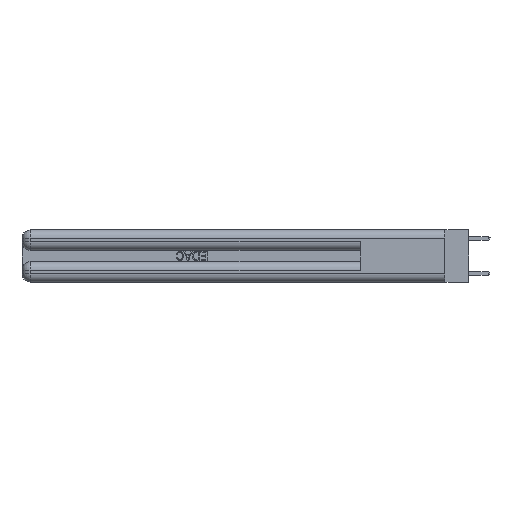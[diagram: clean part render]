
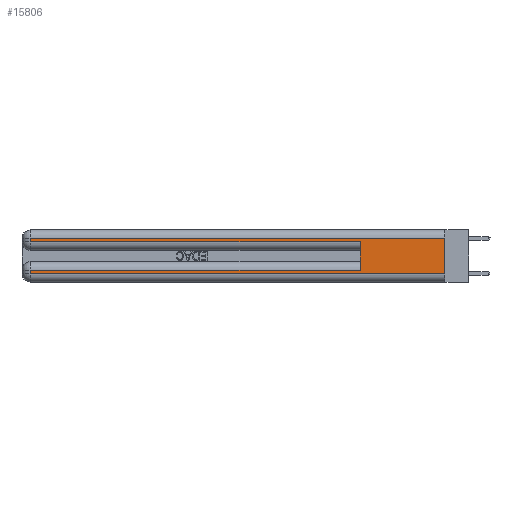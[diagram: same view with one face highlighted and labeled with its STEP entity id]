
A CAD part, left-side view. The second image highlights one B-rep face of the part: STEP entity #15806.
In plain terms, the highlighted planar face has unit normal (-1, 0, 0).
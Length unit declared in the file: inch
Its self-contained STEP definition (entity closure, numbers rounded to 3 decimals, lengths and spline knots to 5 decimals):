
#4 = FACE_OUTER_BOUND ( 'NONE', #20105, .T. ) ;
#513 = LINE ( 'NONE', #12266, #721 ) ;
#721 = VECTOR ( 'NONE', #13948, 39.37008 ) ;
#782 = VERTEX_POINT ( 'NONE', #14683 ) ;
#1270 = VECTOR ( 'NONE', #3273, 39.37008 ) ;
#1611 = DIRECTION ( 'NONE',  ( 0., -1., 0. ) ) ;
#2240 = CARTESIAN_POINT ( 'NONE',  ( 0., 2.94, 0.085 ) ) ;
#3273 = DIRECTION ( 'NONE',  ( 0., 0., -1. ) ) ;
#3475 = LINE ( 'NONE', #22020, #19058 ) ;
#3523 = EDGE_CURVE ( 'NONE', #8082, #11366, #8468, .T. ) ;
#3749 = LINE ( 'NONE', #10762, #4786 ) ;
#4712 = ORIENTED_EDGE ( 'NONE', *, *, #24804, .T. ) ;
#4786 = VECTOR ( 'NONE', #1611, 39.37008 ) ;
#5029 = PLANE ( 'NONE',  #19413 ) ;
#6337 = CARTESIAN_POINT ( 'NONE',  ( 0., 0., 0.37 ) ) ;
#6552 = DIRECTION ( 'NONE',  ( 0., 0., -1. ) ) ;
#6862 = DIRECTION ( 'NONE',  ( 1., 0., 0. ) ) ;
#7354 = VERTEX_POINT ( 'NONE', #7931 ) ;
#7879 = CARTESIAN_POINT ( 'NONE',  ( 0., 0.6, 0.145 ) ) ;
#7931 = CARTESIAN_POINT ( 'NONE',  ( 0., 0.6, 0.085 ) ) ;
#8082 = VERTEX_POINT ( 'NONE', #9407 ) ;
#8468 = LINE ( 'NONE', #6337, #27039 ) ;
#8994 = LINE ( 'NONE', #24951, #11491 ) ;
#9407 = CARTESIAN_POINT ( 'NONE',  ( 0., 0., 0.31 ) ) ;
#9790 = EDGE_CURVE ( 'NONE', #8082, #16026, #15633, .T. ) ;
#9872 = EDGE_CURVE ( 'NONE', #7354, #21179, #513, .T. ) ;
#10762 = CARTESIAN_POINT ( 'NONE',  ( 0., 0., 0.285 ) ) ;
#11071 = CARTESIAN_POINT ( 'NONE',  ( 0., 0., 0.31 ) ) ;
#11366 = VERTEX_POINT ( 'NONE', #11727 ) ;
#11491 = VECTOR ( 'NONE', #6552, 39.37008 ) ;
#11727 = CARTESIAN_POINT ( 'NONE',  ( 0., 0., 0.06 ) ) ;
#11776 = VERTEX_POINT ( 'NONE', #22781 ) ;
#12266 = CARTESIAN_POINT ( 'NONE',  ( 0., 0., 0.085 ) ) ;
#12577 = CARTESIAN_POINT ( 'NONE',  ( 0., 2.94, 0.37 ) ) ;
#13948 = DIRECTION ( 'NONE',  ( 0., 1., 0. ) ) ;
#14317 = DIRECTION ( 'NONE',  ( 0., 0., -1. ) ) ;
#14683 = CARTESIAN_POINT ( 'NONE',  ( 0., 2.94, 0.285 ) ) ;
#14823 = ORIENTED_EDGE ( 'NONE', *, *, #28142, .F. ) ;
#15228 = EDGE_CURVE ( 'NONE', #782, #11776, #3749, .T. ) ;
#15633 = LINE ( 'NONE', #11071, #26981 ) ;
#15806 = ADVANCED_FACE ( 'NONE', ( #4 ), #5029, .F. ) ;
#16026 = VERTEX_POINT ( 'NONE', #22351 ) ;
#17254 = VERTEX_POINT ( 'NONE', #21204 ) ;
#17764 = EDGE_CURVE ( 'NONE', #17254, #11366, #3475, .T. ) ;
#17771 = ORIENTED_EDGE ( 'NONE', *, *, #9790, .T. ) ;
#18200 = EDGE_CURVE ( 'NONE', #21179, #17254, #24121, .T. ) ;
#18457 = CARTESIAN_POINT ( 'NONE',  ( 0., 0., 0.37 ) ) ;
#18653 = ORIENTED_EDGE ( 'NONE', *, *, #17764, .T. ) ;
#18969 = VECTOR ( 'NONE', #26125, 39.37008 ) ;
#19058 = VECTOR ( 'NONE', #24155, 39.37008 ) ;
#19413 = AXIS2_PLACEMENT_3D ( 'NONE', #18457, #6862, #14317 ) ;
#19460 = LINE ( 'NONE', #7879, #18969 ) ;
#19748 = DIRECTION ( 'NONE',  ( 0., 0., -1. ) ) ;
#20105 = EDGE_LOOP ( 'NONE', ( #26529, #17771, #4712, #24531, #14823, #24361, #23951, #18653 ) ) ;
#20347 = DIRECTION ( 'NONE',  ( 0., 1., 0. ) ) ;
#21179 = VERTEX_POINT ( 'NONE', #2240 ) ;
#21204 = CARTESIAN_POINT ( 'NONE',  ( 0., 2.94, 0.06 ) ) ;
#22020 = CARTESIAN_POINT ( 'NONE',  ( 0., 0., 0.06 ) ) ;
#22351 = CARTESIAN_POINT ( 'NONE',  ( 0., 2.94, 0.31 ) ) ;
#22781 = CARTESIAN_POINT ( 'NONE',  ( 0., 0.6, 0.285 ) ) ;
#23951 = ORIENTED_EDGE ( 'NONE', *, *, #18200, .T. ) ;
#24121 = LINE ( 'NONE', #12577, #1270 ) ;
#24155 = DIRECTION ( 'NONE',  ( 0., -1., 0. ) ) ;
#24361 = ORIENTED_EDGE ( 'NONE', *, *, #9872, .T. ) ;
#24531 = ORIENTED_EDGE ( 'NONE', *, *, #15228, .T. ) ;
#24804 = EDGE_CURVE ( 'NONE', #16026, #782, #8994, .T. ) ;
#24951 = CARTESIAN_POINT ( 'NONE',  ( 0., 2.94, 0.37 ) ) ;
#26125 = DIRECTION ( 'NONE',  ( 0., 0., 1. ) ) ;
#26529 = ORIENTED_EDGE ( 'NONE', *, *, #3523, .F. ) ;
#26981 = VECTOR ( 'NONE', #20347, 39.37008 ) ;
#27039 = VECTOR ( 'NONE', #19748, 39.37008 ) ;
#28142 = EDGE_CURVE ( 'NONE', #7354, #11776, #19460, .T. ) ;
